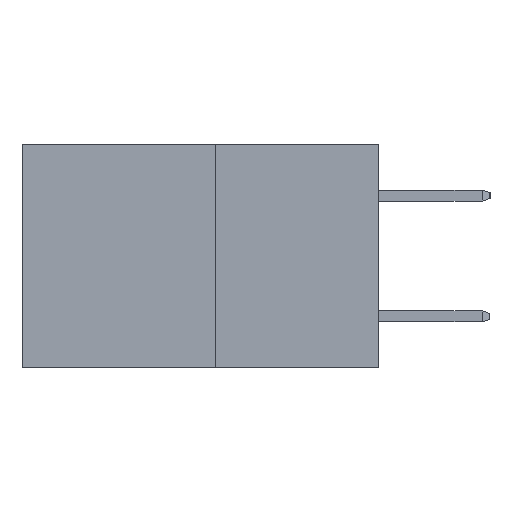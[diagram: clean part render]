
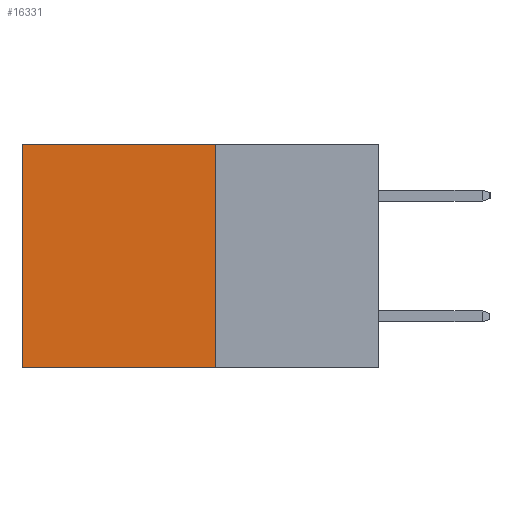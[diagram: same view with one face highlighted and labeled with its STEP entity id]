
A CAD part, left-side view. The second image highlights one B-rep face of the part: STEP entity #16331.
In plain terms, the highlighted planar face has unit normal (-1, 0, 0).
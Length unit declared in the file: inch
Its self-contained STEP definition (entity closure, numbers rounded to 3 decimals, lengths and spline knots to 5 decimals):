
#783 = VECTOR ( 'NONE', #5487, 39.37008 ) ;
#932 = EDGE_CURVE ( 'NONE', #14573, #17637, #12378, .T. ) ;
#1163 = VECTOR ( 'NONE', #9677, 39.37008 ) ;
#1424 = VECTOR ( 'NONE', #2119, 39.37008 ) ;
#1449 = CARTESIAN_POINT ( 'NONE',  ( 0.277, 0.27, 0. ) ) ;
#1642 = EDGE_CURVE ( 'NONE', #14573, #10408, #4947, .T. ) ;
#2119 = DIRECTION ( 'NONE',  ( 0., 0., -1. ) ) ;
#2414 = EDGE_CURVE ( 'NONE', #17637, #6175, #7444, .T. ) ;
#2797 = DIRECTION ( 'NONE',  ( 0., 0., -1. ) ) ;
#4143 = LINE ( 'NONE', #14090, #783 ) ;
#4947 = LINE ( 'NONE', #1449, #1163 ) ;
#5487 = DIRECTION ( 'NONE',  ( 0., 0., -1. ) ) ;
#5922 = ORIENTED_EDGE ( 'NONE', *, *, #932, .F. ) ;
#6175 = VERTEX_POINT ( 'NONE', #14800 ) ;
#7444 = LINE ( 'NONE', #12712, #10792 ) ;
#8507 = CARTESIAN_POINT ( 'NONE',  ( 0.277, 0.27, -0.37 ) ) ;
#8805 = CARTESIAN_POINT ( 'NONE',  ( 0.277, 0.59, 0. ) ) ;
#9428 = ORIENTED_EDGE ( 'NONE', *, *, #2414, .F. ) ;
#9487 = EDGE_LOOP ( 'NONE', ( #14332, #9428, #5922, #17511 ) ) ;
#9524 = FACE_OUTER_BOUND ( 'NONE', #9487, .T. ) ;
#9677 = DIRECTION ( 'NONE',  ( 0., 1., 0. ) ) ;
#10376 = CARTESIAN_POINT ( 'NONE',  ( 0.277, 0.27, 0. ) ) ;
#10408 = VERTEX_POINT ( 'NONE', #8805 ) ;
#10792 = VECTOR ( 'NONE', #11541, 39.37008 ) ;
#11200 = CARTESIAN_POINT ( 'NONE',  ( 0.277, 0.27, -0.37 ) ) ;
#11378 = DIRECTION ( 'NONE',  ( 1., 0., 0. ) ) ;
#11541 = DIRECTION ( 'NONE',  ( 0., 1., 0. ) ) ;
#11946 = AXIS2_PLACEMENT_3D ( 'NONE', #8507, #11378, #2797 ) ;
#12179 = EDGE_CURVE ( 'NONE', #10408, #6175, #4143, .T. ) ;
#12266 = CARTESIAN_POINT ( 'NONE',  ( 0.277, 0.27, -0.37 ) ) ;
#12378 = LINE ( 'NONE', #12266, #1424 ) ;
#12712 = CARTESIAN_POINT ( 'NONE',  ( 0.277, 0.27, -0.37 ) ) ;
#14090 = CARTESIAN_POINT ( 'NONE',  ( 0.277, 0.59, -0.37 ) ) ;
#14195 = PLANE ( 'NONE',  #11946 ) ;
#14332 = ORIENTED_EDGE ( 'NONE', *, *, #12179, .T. ) ;
#14573 = VERTEX_POINT ( 'NONE', #10376 ) ;
#14800 = CARTESIAN_POINT ( 'NONE',  ( 0.277, 0.59, -0.37 ) ) ;
#16331 = ADVANCED_FACE ( 'NONE', ( #9524 ), #14195, .F. ) ;
#17511 = ORIENTED_EDGE ( 'NONE', *, *, #1642, .T. ) ;
#17637 = VERTEX_POINT ( 'NONE', #11200 ) ;
